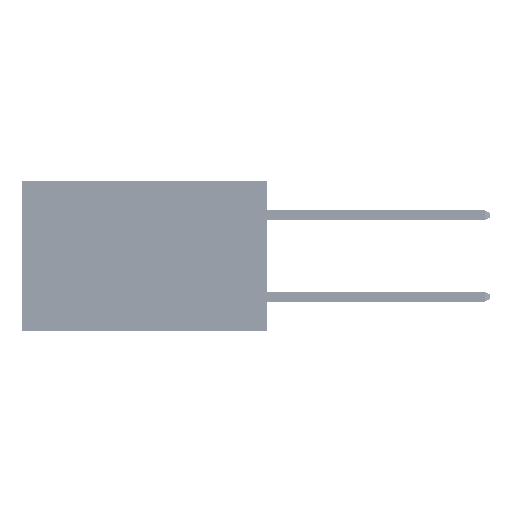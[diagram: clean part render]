
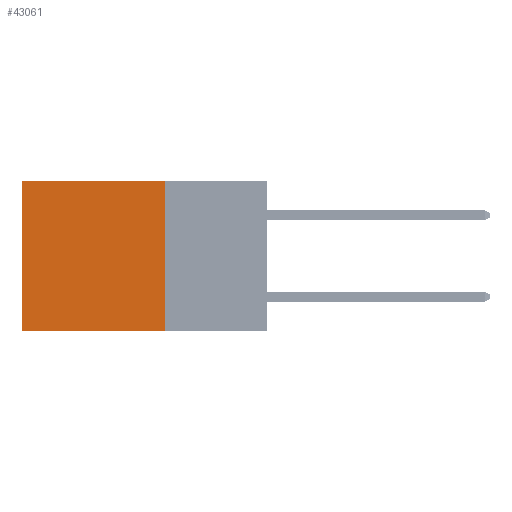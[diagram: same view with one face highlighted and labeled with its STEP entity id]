
A CAD part, left-side view. The second image highlights one B-rep face of the part: STEP entity #43061.
In plain terms, the highlighted planar face has unit normal (-1, 0, 0).
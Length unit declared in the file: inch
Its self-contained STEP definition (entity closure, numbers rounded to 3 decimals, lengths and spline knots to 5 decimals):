
#1199 = ORIENTED_EDGE ( 'NONE', *, *, #49916, .F. ) ;
#3152 = VERTEX_POINT ( 'NONE', #14627 ) ;
#8350 = VECTOR ( 'NONE', #12599, 39.37008 ) ;
#9017 = LINE ( 'NONE', #48011, #8350 ) ;
#9972 = PLANE ( 'NONE',  #35730 ) ;
#10753 = VERTEX_POINT ( 'NONE', #40345 ) ;
#12599 = DIRECTION ( 'NONE',  ( 0., 0., -1. ) ) ;
#14627 = CARTESIAN_POINT ( 'NONE',  ( 0.2875, 0.6, 0. ) ) ;
#16060 = VECTOR ( 'NONE', #34786, 39.37008 ) ;
#19283 = EDGE_LOOP ( 'NONE', ( #49896, #1199, #25449, #21157 ) ) ;
#20021 = EDGE_CURVE ( 'NONE', #10753, #3152, #45464, .T. ) ;
#21157 = ORIENTED_EDGE ( 'NONE', *, *, #20021, .T. ) ;
#22066 = CARTESIAN_POINT ( 'NONE',  ( 0.2875, 0.25, -0.37 ) ) ;
#22802 = CARTESIAN_POINT ( 'NONE',  ( 0.2875, 0.6, 0. ) ) ;
#23291 = LINE ( 'NONE', #22802, #16060 ) ;
#25159 = DIRECTION ( 'NONE',  ( 0., 1., 0. ) ) ;
#25449 = ORIENTED_EDGE ( 'NONE', *, *, #48658, .F. ) ;
#25513 = DIRECTION ( 'NONE',  ( 0., 0., -1. ) ) ;
#28239 = CARTESIAN_POINT ( 'NONE',  ( 0.2875, 0.25, -0.37 ) ) ;
#29025 = VERTEX_POINT ( 'NONE', #22066 ) ;
#29581 = FACE_OUTER_BOUND ( 'NONE', #19283, .T. ) ;
#31338 = DIRECTION ( 'NONE',  ( 0., 1., 0. ) ) ;
#32649 = DIRECTION ( 'NONE',  ( 1., 0., 0. ) ) ;
#34786 = DIRECTION ( 'NONE',  ( 0., 0., -1. ) ) ;
#35411 = LINE ( 'NONE', #28239, #49139 ) ;
#35730 = AXIS2_PLACEMENT_3D ( 'NONE', #45136, #32649, #25513 ) ;
#36879 = CARTESIAN_POINT ( 'NONE',  ( 0.2875, 0.25, 0. ) ) ;
#40345 = CARTESIAN_POINT ( 'NONE',  ( 0.2875, 0.25, 0. ) ) ;
#41021 = EDGE_CURVE ( 'NONE', #3152, #50021, #23291, .T. ) ;
#43061 = ADVANCED_FACE ( 'NONE', ( #29581 ), #9972, .F. ) ;
#45136 = CARTESIAN_POINT ( 'NONE',  ( 0.2875, 0.25, 0. ) ) ;
#45464 = LINE ( 'NONE', #36879, #46204 ) ;
#46204 = VECTOR ( 'NONE', #25159, 39.37008 ) ;
#47383 = CARTESIAN_POINT ( 'NONE',  ( 0.2875, 0.6, -0.37 ) ) ;
#48011 = CARTESIAN_POINT ( 'NONE',  ( 0.2875, 0.25, 0. ) ) ;
#48658 = EDGE_CURVE ( 'NONE', #10753, #29025, #9017, .T. ) ;
#49139 = VECTOR ( 'NONE', #31338, 39.37008 ) ;
#49896 = ORIENTED_EDGE ( 'NONE', *, *, #41021, .T. ) ;
#49916 = EDGE_CURVE ( 'NONE', #29025, #50021, #35411, .T. ) ;
#50021 = VERTEX_POINT ( 'NONE', #47383 ) ;
